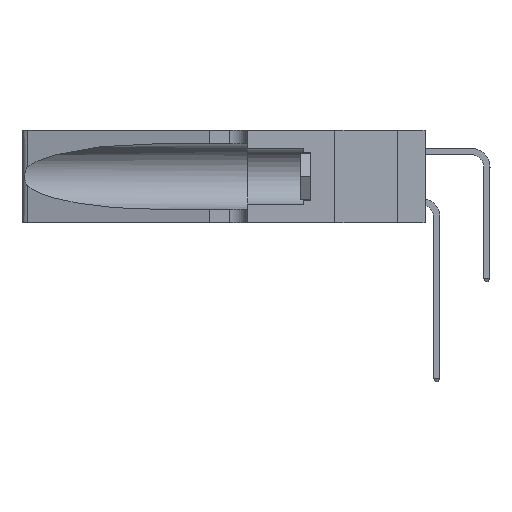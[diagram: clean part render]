
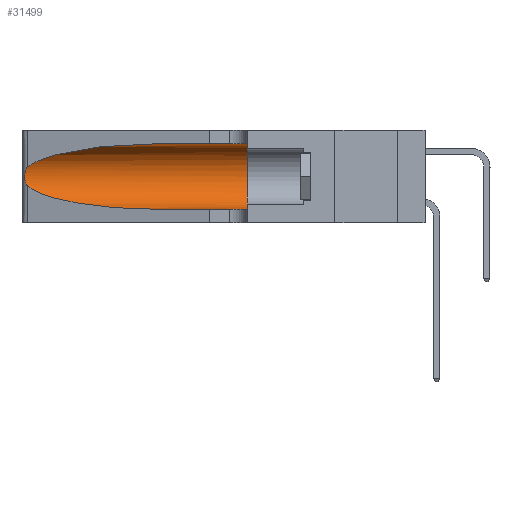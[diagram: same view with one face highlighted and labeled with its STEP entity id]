
A CAD part, left-side view. The second image highlights one B-rep face of the part: STEP entity #31499.
In plain terms, the highlighted cylindrical face has radius 3.308 mm (diameter 6.617 mm), a partial arc.
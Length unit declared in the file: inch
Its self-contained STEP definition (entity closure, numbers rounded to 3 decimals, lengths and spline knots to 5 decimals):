
#2141 = B_SPLINE_CURVE_WITH_KNOTS ( 'NONE', 3,
 ( #33257, #8206, #24460, #15243, #21364, #8999, #39785, #30661, #5879, #27568, #12258, #39915, #27822, #11999 ),
 .UNSPECIFIED., .F., .F.,
 ( 4, 2, 2, 2, 2, 2, 4 ),
 ( 0., 0.00027, 0.00053, 0.00107, 0.0016, 0.00187, 0.00214 ),
 .UNSPECIFIED. ) ;
#3264 = VERTEX_POINT ( 'NONE', #30623 ) ;
#3559 = CYLINDRICAL_SURFACE ( 'NONE', #5989, 0.13025 ) ;
#4578 = VECTOR ( 'NONE', #19811, 39.37008 ) ;
#5777 = CARTESIAN_POINT ( 'NONE',  ( 0.1305, 0.72297, 0.05475 ) ) ;
#5879 = CARTESIAN_POINT ( 'NONE',  ( 0.26017, 1.23833, 0.17102 ) ) ;
#5989 = AXIS2_PLACEMENT_3D ( 'NONE', #24784, #37656, #9191 ) ;
#7485 = VERTEX_POINT ( 'NONE', #19263 ) ;
#8122 = EDGE_CURVE ( 'NONE', #25641, #40103, #38506, .T. ) ;
#8151 = VERTEX_POINT ( 'NONE', #24602 ) ;
#8206 = CARTESIAN_POINT ( 'NONE',  ( 0.25555, 1.22994, 0.2215 ) ) ;
#8491 = ORIENTED_EDGE ( 'NONE', *, *, #17559, .F. ) ;
#8999 = CARTESIAN_POINT ( 'NONE',  ( 0.26018, 1.23835, 0.19895 ) ) ;
#9191 = DIRECTION ( 'NONE',  ( 0., 0., -1. ) ) ;
#9498 = ORIENTED_EDGE ( 'NONE', *, *, #22218, .T. ) ;
#10958 = CARTESIAN_POINT ( 'NONE',  ( 0.1305, 0.35, 0.31525 ) ) ;
#11376 = DIRECTION ( 'NONE',  ( 0., -1., 0. ) ) ;
#11999 = CARTESIAN_POINT ( 'NONE',  ( 0.25487, 1.22718, 0.14631 ) ) ;
#12258 = CARTESIAN_POINT ( 'NONE',  ( 0.25789, 1.23486, 0.15765 ) ) ;
#14838 = EDGE_CURVE ( 'NONE', #31768, #3264, #17447, .T. ) ;
#15002 = CARTESIAN_POINT ( 'NONE',  ( 0.25487, 1.22718, 0.14631 ) ) ;
#15243 = CARTESIAN_POINT ( 'NONE',  ( 0.25787, 1.23484, 0.2124 ) ) ;
#17447 = CIRCLE ( 'NONE', #29151, 0.13025 ) ;
#17559 = EDGE_CURVE ( 'NONE', #25641, #31768, #39989, .T. ) ;
#18386 = CARTESIAN_POINT ( 'NONE',  ( 0.25487, 1.22718, 0.22369 ) ) ;
#18641 = DIRECTION ( 'NONE',  ( 0., 1., 0. ) ) ;
#19263 = CARTESIAN_POINT ( 'NONE',  ( 0.1305, 0.72297, 0.05475 ) ) ;
#19811 = DIRECTION ( 'NONE',  ( 0., -1., 0. ) ) ;
#20209 = CARTESIAN_POINT ( 'NONE',  ( 0.25487, 1.22718, 0.22369 ) ) ;
#21364 = CARTESIAN_POINT ( 'NONE',  ( 0.25854, 1.2359, 0.20912 ) ) ;
#21771 = CARTESIAN_POINT ( 'NONE',  ( 0.2373, 1.15595, 0.28018 ) ) ;
#21893 = CARTESIAN_POINT ( 'NONE',  ( 0.18966, 0.96281, 0.31525 ) ) ;
#22218 = EDGE_CURVE ( 'NONE', #8151, #7485, #39957, .T. ) ;
#22716 = EDGE_LOOP ( 'NONE', ( #33539, #36975, #9498, #31459, #30375, #8491 ) ) ;
#24082 = CARTESIAN_POINT ( 'NONE',  ( 0.18966, 0.96281, 0.05475 ) ) ;
#24460 = CARTESIAN_POINT ( 'NONE',  ( 0.25639, 1.23184, 0.21858 ) ) ;
#24602 = CARTESIAN_POINT ( 'NONE',  ( 0.25487, 1.22718, 0.14631 ) ) ;
#24784 = CARTESIAN_POINT ( 'NONE',  ( 0.1305, 1.61858, 0.185 ) ) ;
#25441 = VECTOR ( 'NONE', #11376, 39.37008 ) ;
#25641 = VERTEX_POINT ( 'NONE', #26218 ) ;
#26218 = CARTESIAN_POINT ( 'NONE',  ( 0.1305, 0.72297, 0.31525 ) ) ;
#26682 = CARTESIAN_POINT ( 'NONE',  ( 0.1305, 1.61858, 0.05475 ) ) ;
#27063 = CARTESIAN_POINT ( 'NONE',  ( 0.2373, 1.15595, 0.08982 ) ) ;
#27568 = CARTESIAN_POINT ( 'NONE',  ( 0.25856, 1.23593, 0.16098 ) ) ;
#27822 = CARTESIAN_POINT ( 'NONE',  ( 0.25555, 1.22993, 0.14849 ) ) ;
#27838 = LINE ( 'NONE', #26682, #25441 ) ;
#29151 = AXIS2_PLACEMENT_3D ( 'NONE', #33932, #18641, #34202 ) ;
#30375 = ORIENTED_EDGE ( 'NONE', *, *, #14838, .F. ) ;
#30623 = CARTESIAN_POINT ( 'NONE',  ( 0.1305, 0.35, 0.05475 ) ) ;
#30661 = CARTESIAN_POINT ( 'NONE',  ( 0.26075, 1.23896, 0.178 ) ) ;
#31459 = ORIENTED_EDGE ( 'NONE', *, *, #39206, .T. ) ;
#31499 = ADVANCED_FACE ( 'NONE', ( #39011 ), #3559, .F. ) ;
#31768 = VERTEX_POINT ( 'NONE', #10958 ) ;
#33257 = CARTESIAN_POINT ( 'NONE',  ( 0.25487, 1.22718, 0.22369 ) ) ;
#33539 = ORIENTED_EDGE ( 'NONE', *, *, #8122, .T. ) ;
#33932 = CARTESIAN_POINT ( 'NONE',  ( 0.1305, 0.35, 0.185 ) ) ;
#34202 = DIRECTION ( 'NONE',  ( 0., 0., 1. ) ) ;
#36926 = CARTESIAN_POINT ( 'NONE',  ( 0.1305, 0.72297, 0.31525 ) ) ;
#36975 = ORIENTED_EDGE ( 'NONE', *, *, #38018, .T. ) ;
#37656 = DIRECTION ( 'NONE',  ( 0., -1., 0. ) ) ;
#38018 = EDGE_CURVE ( 'NONE', #40103, #8151, #2141, .T. ) ;
#38506 =( BOUNDED_CURVE ( )  B_SPLINE_CURVE ( 3, ( #36926, #21893, #21771, #18386 ),
 .UNSPECIFIED., .F., .T. ) 
 B_SPLINE_CURVE_WITH_KNOTS ( ( 4, 4 ),
 ( 1.5708, 2.84003 ),
 .UNSPECIFIED. ) 
 CURVE ( )  GEOMETRIC_REPRESENTATION_ITEM ( )  RATIONAL_B_SPLINE_CURVE ( ( 1., 0.87, 0.87, 1. ) ) 
 REPRESENTATION_ITEM ( '' )  );
#39011 = FACE_OUTER_BOUND ( 'NONE', #22716, .T. ) ;
#39206 = EDGE_CURVE ( 'NONE', #7485, #3264, #27838, .T. ) ;
#39314 = CARTESIAN_POINT ( 'NONE',  ( 0.1305, 1.61858, 0.31525 ) ) ;
#39785 = CARTESIAN_POINT ( 'NONE',  ( 0.26075, 1.23896, 0.19203 ) ) ;
#39915 = CARTESIAN_POINT ( 'NONE',  ( 0.25639, 1.23186, 0.15144 ) ) ;
#39957 =( BOUNDED_CURVE ( )  B_SPLINE_CURVE ( 3, ( #15002, #27063, #24082, #5777 ),
 .UNSPECIFIED., .F., .F. ) 
 B_SPLINE_CURVE_WITH_KNOTS ( ( 4, 4 ),
 ( 3.44316, 4.71239 ),
 .UNSPECIFIED. ) 
 CURVE ( )  GEOMETRIC_REPRESENTATION_ITEM ( )  RATIONAL_B_SPLINE_CURVE ( ( 1., 0.87, 0.87, 1. ) ) 
 REPRESENTATION_ITEM ( '' )  );
#39989 = LINE ( 'NONE', #39314, #4578 ) ;
#40103 = VERTEX_POINT ( 'NONE', #20209 ) ;
